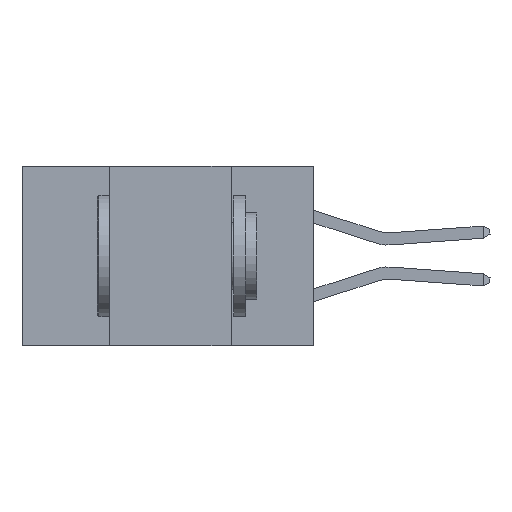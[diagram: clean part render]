
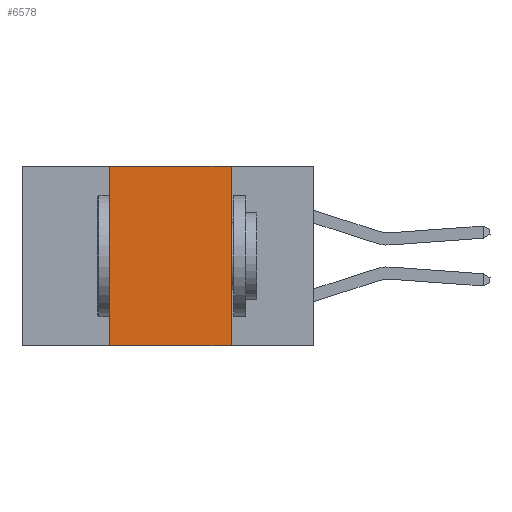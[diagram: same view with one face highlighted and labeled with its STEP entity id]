
A CAD part, left-side view. The second image highlights one B-rep face of the part: STEP entity #6578.
In plain terms, the highlighted planar face has unit normal (-1, 0, 0).
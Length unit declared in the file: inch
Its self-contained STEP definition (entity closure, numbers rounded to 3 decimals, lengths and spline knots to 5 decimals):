
#956 = FACE_OUTER_BOUND ( 'NONE', #1428, .T. ) ;
#1428 = EDGE_LOOP ( 'NONE', ( #14919, #15817, #19016, #16487 ) ) ;
#1649 = LINE ( 'NONE', #9037, #8115 ) ;
#1685 = DIRECTION ( 'NONE',  ( 0., -1., 0. ) ) ;
#2012 = LINE ( 'NONE', #11195, #20217 ) ;
#4027 = PLANE ( 'NONE',  #28658 ) ;
#4167 = DIRECTION ( 'NONE',  ( 0., 0., -1. ) ) ;
#6495 = CARTESIAN_POINT ( 'NONE',  ( 0., 0.6, 0. ) ) ;
#6578 = ADVANCED_FACE ( 'NONE', ( #956 ), #4027, .F. ) ;
#7168 = VERTEX_POINT ( 'NONE', #18316 ) ;
#7645 = LINE ( 'NONE', #28974, #13944 ) ;
#8091 = CARTESIAN_POINT ( 'NONE',  ( 0., 0.17, 0. ) ) ;
#8115 = VECTOR ( 'NONE', #11307, 39.37008 ) ;
#8932 = DIRECTION ( 'NONE',  ( 1., 0., 0. ) ) ;
#9037 = CARTESIAN_POINT ( 'NONE',  ( 0., 0.6, -0.37 ) ) ;
#10520 = VERTEX_POINT ( 'NONE', #8091 ) ;
#11195 = CARTESIAN_POINT ( 'NONE',  ( 0., 0.6, 0. ) ) ;
#11307 = DIRECTION ( 'NONE',  ( 0., -1., 0. ) ) ;
#11619 = VERTEX_POINT ( 'NONE', #13535 ) ;
#13102 = VERTEX_POINT ( 'NONE', #21418 ) ;
#13535 = CARTESIAN_POINT ( 'NONE',  ( 0., 0.17, -0.37 ) ) ;
#13944 = VECTOR ( 'NONE', #22202, 39.37008 ) ;
#14687 = LINE ( 'NONE', #16054, #21639 ) ;
#14919 = ORIENTED_EDGE ( 'NONE', *, *, #23195, .F. ) ;
#15817 = ORIENTED_EDGE ( 'NONE', *, *, #20970, .F. ) ;
#16054 = CARTESIAN_POINT ( 'NONE',  ( 0., 0.17, 0. ) ) ;
#16129 = EDGE_CURVE ( 'NONE', #7168, #11619, #1649, .T. ) ;
#16487 = ORIENTED_EDGE ( 'NONE', *, *, #16129, .T. ) ;
#18316 = CARTESIAN_POINT ( 'NONE',  ( 0., 0.42, -0.37 ) ) ;
#19016 = ORIENTED_EDGE ( 'NONE', *, *, #29592, .F. ) ;
#20217 = VECTOR ( 'NONE', #1685, 39.37008 ) ;
#20970 = EDGE_CURVE ( 'NONE', #13102, #10520, #2012, .T. ) ;
#21418 = CARTESIAN_POINT ( 'NONE',  ( 0., 0.42, 0. ) ) ;
#21639 = VECTOR ( 'NONE', #4167, 39.37008 ) ;
#22202 = DIRECTION ( 'NONE',  ( 0., 0., 1. ) ) ;
#23195 = EDGE_CURVE ( 'NONE', #10520, #11619, #14687, .T. ) ;
#25281 = DIRECTION ( 'NONE',  ( 0., 0., -1. ) ) ;
#28658 = AXIS2_PLACEMENT_3D ( 'NONE', #6495, #8932, #25281 ) ;
#28974 = CARTESIAN_POINT ( 'NONE',  ( 0., 0.42, 0. ) ) ;
#29592 = EDGE_CURVE ( 'NONE', #7168, #13102, #7645, .T. ) ;
